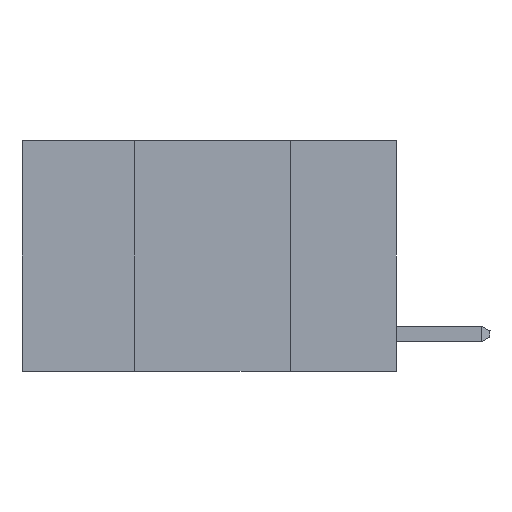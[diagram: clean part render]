
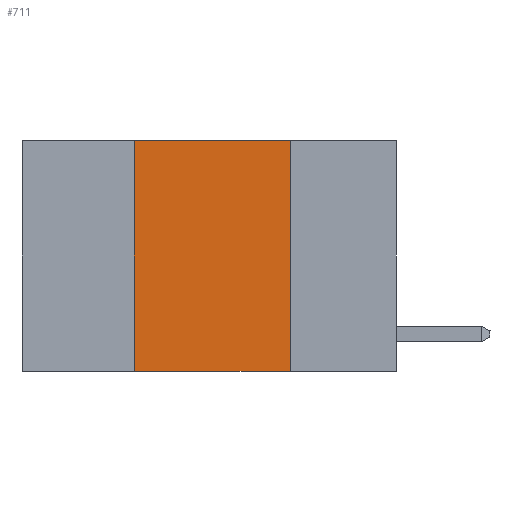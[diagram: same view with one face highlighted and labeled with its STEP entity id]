
A CAD part, left-side view. The second image highlights one B-rep face of the part: STEP entity #711.
In plain terms, the highlighted planar face has unit normal (-1, 0, 0).
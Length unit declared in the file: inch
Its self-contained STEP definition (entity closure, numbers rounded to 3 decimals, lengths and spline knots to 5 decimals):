
#22 = VECTOR ( 'NONE', #23404, 39.37008 ) ;
#503 = CARTESIAN_POINT ( 'NONE',  ( 0., 0.42, -0.37 ) ) ;
#605 = EDGE_CURVE ( 'NONE', #18038, #7117, #14062, .T. ) ;
#711 = ADVANCED_FACE ( 'NONE', ( #26654 ), #23594, .F. ) ;
#1599 = VECTOR ( 'NONE', #7266, 39.37008 ) ;
#2265 = LINE ( 'NONE', #26936, #1599 ) ;
#2544 = EDGE_CURVE ( 'NONE', #21006, #10197, #9198, .T. ) ;
#3544 = ORIENTED_EDGE ( 'NONE', *, *, #2544, .T. ) ;
#6826 = EDGE_CURVE ( 'NONE', #21006, #18038, #7461, .T. ) ;
#7117 = VERTEX_POINT ( 'NONE', #16454 ) ;
#7266 = DIRECTION ( 'NONE',  ( 0., 0., -1. ) ) ;
#7461 = LINE ( 'NONE', #14778, #18381 ) ;
#8169 = CARTESIAN_POINT ( 'NONE',  ( 0., 0.6, -0.37 ) ) ;
#8309 = EDGE_CURVE ( 'NONE', #7117, #10197, #2265, .T. ) ;
#9198 = LINE ( 'NONE', #8169, #22 ) ;
#10197 = VERTEX_POINT ( 'NONE', #23180 ) ;
#10371 = ORIENTED_EDGE ( 'NONE', *, *, #605, .F. ) ;
#10542 = DIRECTION ( 'NONE',  ( 0., 0., -1. ) ) ;
#10874 = ORIENTED_EDGE ( 'NONE', *, *, #6826, .F. ) ;
#12489 = AXIS2_PLACEMENT_3D ( 'NONE', #12804, #28056, #10542 ) ;
#12804 = CARTESIAN_POINT ( 'NONE',  ( 0., 0.6, 0. ) ) ;
#13083 = ORIENTED_EDGE ( 'NONE', *, *, #8309, .F. ) ;
#14062 = LINE ( 'NONE', #25387, #25627 ) ;
#14688 = DIRECTION ( 'NONE',  ( 0., 0., 1. ) ) ;
#14778 = CARTESIAN_POINT ( 'NONE',  ( 0., 0.42, 0. ) ) ;
#16454 = CARTESIAN_POINT ( 'NONE',  ( 0., 0.17, 0. ) ) ;
#16646 = DIRECTION ( 'NONE',  ( 0., -1., 0. ) ) ;
#17091 = EDGE_LOOP ( 'NONE', ( #13083, #10371, #10874, #3544 ) ) ;
#18038 = VERTEX_POINT ( 'NONE', #22365 ) ;
#18381 = VECTOR ( 'NONE', #14688, 39.37008 ) ;
#21006 = VERTEX_POINT ( 'NONE', #503 ) ;
#22365 = CARTESIAN_POINT ( 'NONE',  ( 0., 0.42, 0. ) ) ;
#23180 = CARTESIAN_POINT ( 'NONE',  ( 0., 0.17, -0.37 ) ) ;
#23404 = DIRECTION ( 'NONE',  ( 0., -1., 0. ) ) ;
#23594 = PLANE ( 'NONE',  #12489 ) ;
#25387 = CARTESIAN_POINT ( 'NONE',  ( 0., 0.6, 0. ) ) ;
#25627 = VECTOR ( 'NONE', #16646, 39.37008 ) ;
#26654 = FACE_OUTER_BOUND ( 'NONE', #17091, .T. ) ;
#26936 = CARTESIAN_POINT ( 'NONE',  ( 0., 0.17, 0. ) ) ;
#28056 = DIRECTION ( 'NONE',  ( 1., 0., 0. ) ) ;
